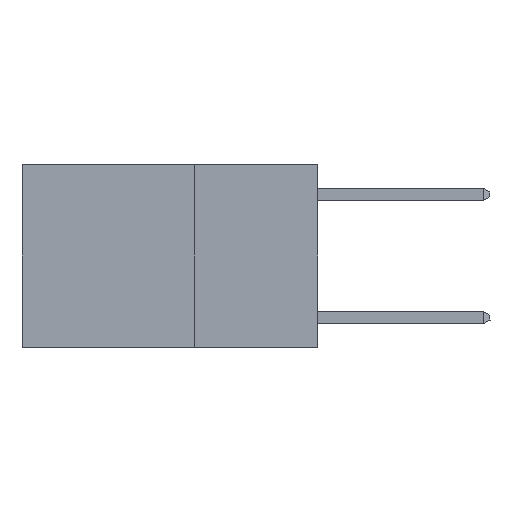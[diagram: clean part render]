
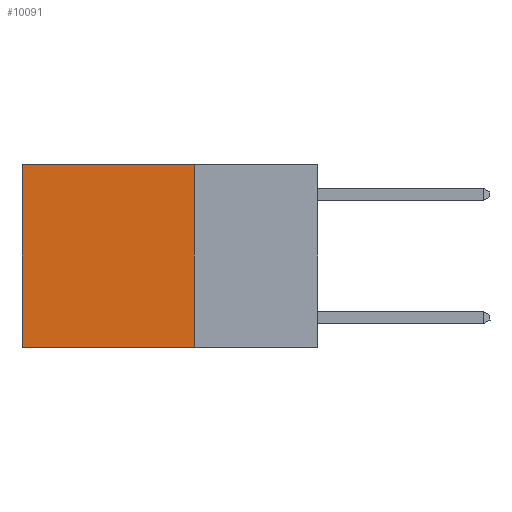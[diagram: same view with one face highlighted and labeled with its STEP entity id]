
A CAD part, left-side view. The second image highlights one B-rep face of the part: STEP entity #10091.
In plain terms, the highlighted planar face has unit normal (-1, 0, 0).
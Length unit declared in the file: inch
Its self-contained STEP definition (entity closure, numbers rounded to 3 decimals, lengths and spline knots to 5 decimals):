
#587 = DIRECTION ( 'NONE',  ( 0., 1., 0. ) ) ;
#1189 = DIRECTION ( 'NONE',  ( 1., 0., 0. ) ) ;
#1223 = DIRECTION ( 'NONE',  ( 0., 1., 0. ) ) ;
#1880 = EDGE_CURVE ( 'NONE', #4348, #11480, #3306, .T. ) ;
#2213 = CARTESIAN_POINT ( 'NONE',  ( 0.2625, 0.6, 0. ) ) ;
#2284 = CARTESIAN_POINT ( 'NONE',  ( 0.2625, 0.25, -0.37 ) ) ;
#3306 = LINE ( 'NONE', #12398, #3325 ) ;
#3325 = VECTOR ( 'NONE', #5591, 39.37008 ) ;
#3543 = ORIENTED_EDGE ( 'NONE', *, *, #10333, .T. ) ;
#3556 = VECTOR ( 'NONE', #587, 39.37008 ) ;
#4288 = ORIENTED_EDGE ( 'NONE', *, *, #1880, .F. ) ;
#4348 = VERTEX_POINT ( 'NONE', #12197 ) ;
#4488 = ORIENTED_EDGE ( 'NONE', *, *, #9009, .F. ) ;
#5298 = CARTESIAN_POINT ( 'NONE',  ( 0.2625, 0.6, -0.37 ) ) ;
#5591 = DIRECTION ( 'NONE',  ( 0., 0., -1. ) ) ;
#5605 = FACE_OUTER_BOUND ( 'NONE', #8910, .T. ) ;
#5617 = LINE ( 'NONE', #12185, #12790 ) ;
#6105 = VERTEX_POINT ( 'NONE', #2213 ) ;
#6183 = VERTEX_POINT ( 'NONE', #5298 ) ;
#6220 = CARTESIAN_POINT ( 'NONE',  ( 0.2625, 0.25, -0.37 ) ) ;
#7128 = PLANE ( 'NONE',  #11124 ) ;
#7540 = CARTESIAN_POINT ( 'NONE',  ( 0.2625, 0.25, 0. ) ) ;
#7782 = VECTOR ( 'NONE', #1223, 39.37008 ) ;
#8068 = CARTESIAN_POINT ( 'NONE',  ( 0.2625, 0.25, 0. ) ) ;
#8110 = DIRECTION ( 'NONE',  ( 0., 0., -1. ) ) ;
#8829 = LINE ( 'NONE', #7540, #3556 ) ;
#8910 = EDGE_LOOP ( 'NONE', ( #12745, #4488, #4288, #3543 ) ) ;
#9009 = EDGE_CURVE ( 'NONE', #11480, #6183, #12660, .T. ) ;
#9295 = DIRECTION ( 'NONE',  ( 0., 0., -1. ) ) ;
#9642 = EDGE_CURVE ( 'NONE', #6105, #6183, #5617, .T. ) ;
#10091 = ADVANCED_FACE ( 'NONE', ( #5605 ), #7128, .F. ) ;
#10333 = EDGE_CURVE ( 'NONE', #4348, #6105, #8829, .T. ) ;
#11124 = AXIS2_PLACEMENT_3D ( 'NONE', #8068, #1189, #8110 ) ;
#11480 = VERTEX_POINT ( 'NONE', #2284 ) ;
#12185 = CARTESIAN_POINT ( 'NONE',  ( 0.2625, 0.6, 0. ) ) ;
#12197 = CARTESIAN_POINT ( 'NONE',  ( 0.2625, 0.25, 0. ) ) ;
#12398 = CARTESIAN_POINT ( 'NONE',  ( 0.2625, 0.25, 0. ) ) ;
#12660 = LINE ( 'NONE', #6220, #7782 ) ;
#12745 = ORIENTED_EDGE ( 'NONE', *, *, #9642, .T. ) ;
#12790 = VECTOR ( 'NONE', #9295, 39.37008 ) ;
